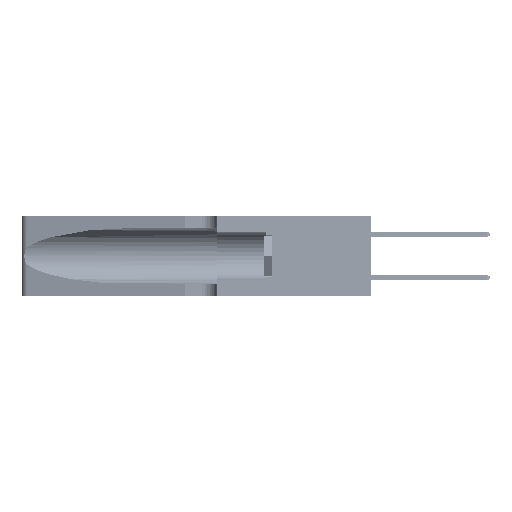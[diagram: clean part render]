
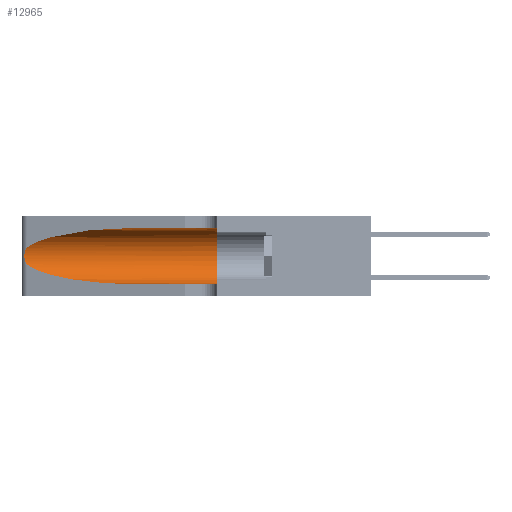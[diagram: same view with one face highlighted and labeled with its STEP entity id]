
A CAD part, left-side view. The second image highlights one B-rep face of the part: STEP entity #12965.
In plain terms, the highlighted cylindrical face has radius 3.308 mm (diameter 6.617 mm), a partial arc.
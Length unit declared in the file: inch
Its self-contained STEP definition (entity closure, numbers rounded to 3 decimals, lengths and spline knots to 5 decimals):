
#2062 = DIRECTION ( 'NONE',  ( 0., -1., 0. ) ) ;
#2627 = CYLINDRICAL_SURFACE ( 'NONE', #41711, 0.13025 ) ;
#3727 = VECTOR ( 'NONE', #2062, 39.37008 ) ;
#3773 = VERTEX_POINT ( 'NONE', #11311 ) ;
#4897 = CARTESIAN_POINT ( 'NONE',  ( 0.25487, 1.22718, 0.22369 ) ) ;
#5213 = CARTESIAN_POINT ( 'NONE',  ( 0.25639, 1.23186, 0.15144 ) ) ;
#7618 = AXIS2_PLACEMENT_3D ( 'NONE', #12089, #23023, #46087 ) ;
#8145 = CARTESIAN_POINT ( 'NONE',  ( 0.1305, 0.72297, 0.05475 ) ) ;
#8659 = CARTESIAN_POINT ( 'NONE',  ( 0.1305, 1.61858, 0.185 ) ) ;
#8856 = CARTESIAN_POINT ( 'NONE',  ( 0.25555, 1.22993, 0.14849 ) ) ;
#11311 = CARTESIAN_POINT ( 'NONE',  ( 0.1305, 0.35, 0.05475 ) ) ;
#11815 = CARTESIAN_POINT ( 'NONE',  ( 0.18966, 0.96281, 0.05475 ) ) ;
#12089 = CARTESIAN_POINT ( 'NONE',  ( 0.1305, 0.35, 0.185 ) ) ;
#12204 = CARTESIAN_POINT ( 'NONE',  ( 0.1305, 0.35, 0.31525 ) ) ;
#12480 = CARTESIAN_POINT ( 'NONE',  ( 0.25487, 1.22718, 0.14631 ) ) ;
#12549 = VERTEX_POINT ( 'NONE', #47411 ) ;
#12702 = CARTESIAN_POINT ( 'NONE',  ( 0.25555, 1.22994, 0.2215 ) ) ;
#12965 = ADVANCED_FACE ( 'NONE', ( #15592 ), #2627, .F. ) ;
#12966 = VECTOR ( 'NONE', #39167, 39.37008 ) ;
#13135 = EDGE_CURVE ( 'NONE', #44250, #3773, #41594, .T. ) ;
#13641 = ORIENTED_EDGE ( 'NONE', *, *, #20006, .T. ) ;
#14095 = ORIENTED_EDGE ( 'NONE', *, *, #44867, .T. ) ;
#15592 = FACE_OUTER_BOUND ( 'NONE', #18507, .T. ) ;
#16352 = CARTESIAN_POINT ( 'NONE',  ( 0.1305, 1.61858, 0.31525 ) ) ;
#16587 = ORIENTED_EDGE ( 'NONE', *, *, #25133, .T. ) ;
#17184 = CARTESIAN_POINT ( 'NONE',  ( 0.1305, 0.72297, 0.31525 ) ) ;
#17527 = CARTESIAN_POINT ( 'NONE',  ( 0.1305, 0.72297, 0.05475 ) ) ;
#18507 = EDGE_LOOP ( 'NONE', ( #14095, #16587, #13641, #35120, #22656, #27344 ) ) ;
#20006 = EDGE_CURVE ( 'NONE', #12549, #44250, #47714, .T. ) ;
#20026 = LINE ( 'NONE', #16352, #12966 ) ;
#20131 = CARTESIAN_POINT ( 'NONE',  ( 0.26075, 1.23896, 0.19203 ) ) ;
#20914 = CARTESIAN_POINT ( 'NONE',  ( 0.1305, 1.61858, 0.05475 ) ) ;
#21383 = B_SPLINE_CURVE_WITH_KNOTS ( 'NONE', 3,
 ( #4897, #12702, #28239, #42753, #24139, #39127, #20131, #23971, #46541, #27736, #31537, #5213, #8856, #42906 ),
 .UNSPECIFIED., .F., .F.,
 ( 4, 2, 2, 2, 2, 2, 4 ),
 ( 0., 0.00027, 0.00053, 0.00107, 0.0016, 0.00187, 0.00214 ),
 .UNSPECIFIED. ) ;
#22656 = ORIENTED_EDGE ( 'NONE', *, *, #28429, .F. ) ;
#23023 = DIRECTION ( 'NONE',  ( 0., 1., 0. ) ) ;
#23509 = VERTEX_POINT ( 'NONE', #42040 ) ;
#23971 = CARTESIAN_POINT ( 'NONE',  ( 0.26075, 1.23896, 0.178 ) ) ;
#24139 = CARTESIAN_POINT ( 'NONE',  ( 0.25854, 1.2359, 0.20912 ) ) ;
#25133 = EDGE_CURVE ( 'NONE', #23509, #12549, #21383, .T. ) ;
#26515 =( BOUNDED_CURVE ( )  B_SPLINE_CURVE ( 3, ( #39472, #39958, #43425, #32224 ),
 .UNSPECIFIED., .F., .F. ) 
 B_SPLINE_CURVE_WITH_KNOTS ( ( 4, 4 ),
 ( 1.5708, 2.84003 ),
 .UNSPECIFIED. ) 
 CURVE ( )  GEOMETRIC_REPRESENTATION_ITEM ( )  RATIONAL_B_SPLINE_CURVE ( ( 1., 0.87, 0.87, 1. ) ) 
 REPRESENTATION_ITEM ( '' )  );
#27344 = ORIENTED_EDGE ( 'NONE', *, *, #33107, .F. ) ;
#27736 = CARTESIAN_POINT ( 'NONE',  ( 0.25856, 1.23593, 0.16098 ) ) ;
#28239 = CARTESIAN_POINT ( 'NONE',  ( 0.25639, 1.23184, 0.21858 ) ) ;
#28429 = EDGE_CURVE ( 'NONE', #30799, #3773, #31709, .T. ) ;
#30799 = VERTEX_POINT ( 'NONE', #12204 ) ;
#30804 = CARTESIAN_POINT ( 'NONE',  ( 0.2373, 1.15595, 0.08982 ) ) ;
#31537 = CARTESIAN_POINT ( 'NONE',  ( 0.25789, 1.23486, 0.15765 ) ) ;
#31709 = CIRCLE ( 'NONE', #7618, 0.13025 ) ;
#32224 = CARTESIAN_POINT ( 'NONE',  ( 0.25487, 1.22718, 0.22369 ) ) ;
#33107 = EDGE_CURVE ( 'NONE', #38800, #30799, #20026, .T. ) ;
#35120 = ORIENTED_EDGE ( 'NONE', *, *, #13135, .T. ) ;
#38585 = DIRECTION ( 'NONE',  ( 0., 0., -1. ) ) ;
#38800 = VERTEX_POINT ( 'NONE', #17184 ) ;
#39127 = CARTESIAN_POINT ( 'NONE',  ( 0.26018, 1.23835, 0.19895 ) ) ;
#39167 = DIRECTION ( 'NONE',  ( 0., -1., 0. ) ) ;
#39472 = CARTESIAN_POINT ( 'NONE',  ( 0.1305, 0.72297, 0.31525 ) ) ;
#39958 = CARTESIAN_POINT ( 'NONE',  ( 0.18966, 0.96281, 0.31525 ) ) ;
#41594 = LINE ( 'NONE', #20914, #3727 ) ;
#41711 = AXIS2_PLACEMENT_3D ( 'NONE', #8659, #42377, #38585 ) ;
#42040 = CARTESIAN_POINT ( 'NONE',  ( 0.25487, 1.22718, 0.22369 ) ) ;
#42377 = DIRECTION ( 'NONE',  ( 0., -1., 0. ) ) ;
#42753 = CARTESIAN_POINT ( 'NONE',  ( 0.25787, 1.23484, 0.2124 ) ) ;
#42906 = CARTESIAN_POINT ( 'NONE',  ( 0.25487, 1.22718, 0.14631 ) ) ;
#43425 = CARTESIAN_POINT ( 'NONE',  ( 0.2373, 1.15595, 0.28018 ) ) ;
#44250 = VERTEX_POINT ( 'NONE', #17527 ) ;
#44867 = EDGE_CURVE ( 'NONE', #38800, #23509, #26515, .T. ) ;
#46087 = DIRECTION ( 'NONE',  ( 0., 0., 1. ) ) ;
#46541 = CARTESIAN_POINT ( 'NONE',  ( 0.26017, 1.23833, 0.17102 ) ) ;
#47411 = CARTESIAN_POINT ( 'NONE',  ( 0.25487, 1.22718, 0.14631 ) ) ;
#47714 =( BOUNDED_CURVE ( )  B_SPLINE_CURVE ( 3, ( #12480, #30804, #11815, #8145 ),
 .UNSPECIFIED., .F., .F. ) 
 B_SPLINE_CURVE_WITH_KNOTS ( ( 4, 4 ),
 ( 3.44316, 4.71239 ),
 .UNSPECIFIED. ) 
 CURVE ( )  GEOMETRIC_REPRESENTATION_ITEM ( )  RATIONAL_B_SPLINE_CURVE ( ( 1., 0.87, 0.87, 1. ) ) 
 REPRESENTATION_ITEM ( '' )  );
